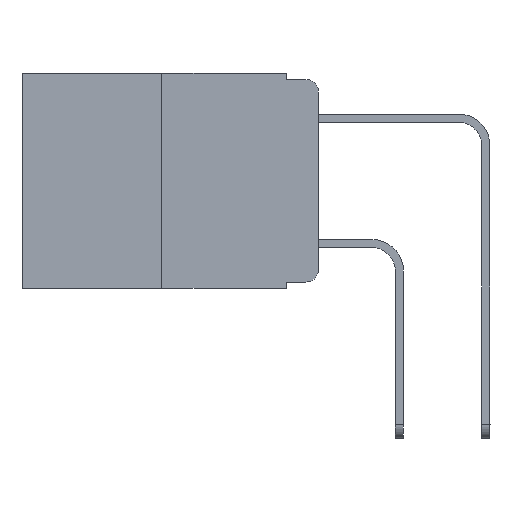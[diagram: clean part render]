
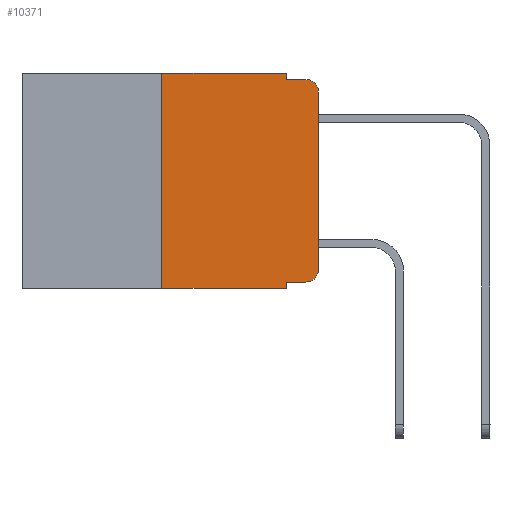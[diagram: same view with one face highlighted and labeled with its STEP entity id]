
A CAD part, left-side view. The second image highlights one B-rep face of the part: STEP entity #10371.
In plain terms, the highlighted planar face has unit normal (-1, 0, 0).
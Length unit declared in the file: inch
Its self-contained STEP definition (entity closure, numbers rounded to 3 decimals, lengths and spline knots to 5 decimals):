
#50 = CARTESIAN_POINT ( 'NONE',  ( 0., 0.02, -0.333 ) ) ;
#106 = DIRECTION ( 'NONE',  ( 0., 0., 1. ) ) ;
#331 = DIRECTION ( 'NONE',  ( 0., 0., -1. ) ) ;
#519 = LINE ( 'NONE', #2161, #13176 ) ;
#569 = DIRECTION ( 'NONE',  ( -1., 0., 0. ) ) ;
#697 = ORIENTED_EDGE ( 'NONE', *, *, #8291, .T. ) ;
#774 = LINE ( 'NONE', #5736, #8462 ) ;
#826 = ORIENTED_EDGE ( 'NONE', *, *, #14375, .T. ) ;
#1158 = EDGE_CURVE ( 'NONE', #8993, #12565, #5526, .T. ) ;
#1278 = ORIENTED_EDGE ( 'NONE', *, *, #1158, .F. ) ;
#1641 = PLANE ( 'NONE',  #4406 ) ;
#1923 = CARTESIAN_POINT ( 'NONE',  ( 0., 0.051, -0.333 ) ) ;
#2083 = VERTEX_POINT ( 'NONE', #13376 ) ;
#2118 = EDGE_CURVE ( 'NONE', #4404, #9830, #774, .T. ) ;
#2161 = CARTESIAN_POINT ( 'NONE',  ( 0., 0.473, -0.343 ) ) ;
#2166 = CARTESIAN_POINT ( 'NONE',  ( 0., 0.473, 0. ) ) ;
#2220 = ORIENTED_EDGE ( 'NONE', *, *, #2118, .F. ) ;
#2834 = EDGE_CURVE ( 'NONE', #12487, #8993, #9660, .T. ) ;
#2847 = EDGE_CURVE ( 'NONE', #10717, #12487, #7281, .T. ) ;
#3379 = CARTESIAN_POINT ( 'NONE',  ( 0., 0.051, 0. ) ) ;
#3672 = VECTOR ( 'NONE', #331, 39.37008 ) ;
#4078 = ORIENTED_EDGE ( 'NONE', *, *, #11253, .T. ) ;
#4216 = DIRECTION ( 'NONE',  ( 0., 0., -1. ) ) ;
#4354 = CARTESIAN_POINT ( 'NONE',  ( 0., 0.02, -0.313 ) ) ;
#4358 = CARTESIAN_POINT ( 'NONE',  ( 0., 0.051, 0. ) ) ;
#4399 = DIRECTION ( 'NONE',  ( 0., 0., -1. ) ) ;
#4404 = VERTEX_POINT ( 'NONE', #1923 ) ;
#4406 = AXIS2_PLACEMENT_3D ( 'NONE', #11532, #14225, #10143 ) ;
#4450 = CARTESIAN_POINT ( 'NONE',  ( 0., 0.051, -0.01 ) ) ;
#4464 = VECTOR ( 'NONE', #14658, 39.37008 ) ;
#4516 = EDGE_CURVE ( 'NONE', #13193, #6578, #13518, .T. ) ;
#4558 = LINE ( 'NONE', #13358, #4464 ) ;
#4631 = ORIENTED_EDGE ( 'NONE', *, *, #2847, .F. ) ;
#4706 = VECTOR ( 'NONE', #106, 39.37008 ) ;
#4885 = DIRECTION ( 'NONE',  ( 0., 0., 1. ) ) ;
#5056 = LINE ( 'NONE', #14007, #4706 ) ;
#5526 = LINE ( 'NONE', #4358, #3672 ) ;
#5600 = ORIENTED_EDGE ( 'NONE', *, *, #2834, .F. ) ;
#5615 = DIRECTION ( 'NONE',  ( 0., 0., -1. ) ) ;
#5736 = CARTESIAN_POINT ( 'NONE',  ( 0., 0.051, 0. ) ) ;
#5893 = VECTOR ( 'NONE', #5963, 39.37008 ) ;
#5963 = DIRECTION ( 'NONE',  ( 0., -1., 0. ) ) ;
#6080 = CARTESIAN_POINT ( 'NONE',  ( 0., 0.25, -0.343 ) ) ;
#6578 = VERTEX_POINT ( 'NONE', #12241 ) ;
#7051 = CARTESIAN_POINT ( 'NONE',  ( 0., 0.051, -0.343 ) ) ;
#7200 = DIRECTION ( 'NONE',  ( 0., -1., 0. ) ) ;
#7281 = LINE ( 'NONE', #8525, #16122 ) ;
#7855 = EDGE_LOOP ( 'NONE', ( #4078, #7937, #10215, #1278, #5600, #4631, #697, #2220, #10686, #826 ) ) ;
#7915 = CIRCLE ( 'NONE', #11060, 0.02 ) ;
#7937 = ORIENTED_EDGE ( 'NONE', *, *, #4516, .T. ) ;
#8265 = DIRECTION ( 'NONE',  ( -1., 0., 0. ) ) ;
#8291 = EDGE_CURVE ( 'NONE', #10717, #9830, #519, .T. ) ;
#8328 = EDGE_CURVE ( 'NONE', #4404, #9976, #4558, .T. ) ;
#8394 = VECTOR ( 'NONE', #10723, 39.37008 ) ;
#8462 = VECTOR ( 'NONE', #4399, 39.37008 ) ;
#8525 = CARTESIAN_POINT ( 'NONE',  ( 0., 0.25, 0. ) ) ;
#8993 = VERTEX_POINT ( 'NONE', #3379 ) ;
#9660 = LINE ( 'NONE', #2166, #5893 ) ;
#9830 = VERTEX_POINT ( 'NONE', #7051 ) ;
#9976 = VERTEX_POINT ( 'NONE', #50 ) ;
#10143 = DIRECTION ( 'NONE',  ( 0., 0., -1. ) ) ;
#10215 = ORIENTED_EDGE ( 'NONE', *, *, #11392, .F. ) ;
#10371 = ADVANCED_FACE ( 'NONE', ( #12683 ), #1641, .F. ) ;
#10686 = ORIENTED_EDGE ( 'NONE', *, *, #8328, .T. ) ;
#10717 = VERTEX_POINT ( 'NONE', #6080 ) ;
#10723 = DIRECTION ( 'NONE',  ( 0., -1., 0. ) ) ;
#10873 = CARTESIAN_POINT ( 'NONE',  ( 0., 0., -0.03 ) ) ;
#11060 = AXIS2_PLACEMENT_3D ( 'NONE', #4354, #569, #5615 ) ;
#11253 = EDGE_CURVE ( 'NONE', #2083, #13193, #5056, .T. ) ;
#11392 = EDGE_CURVE ( 'NONE', #12565, #6578, #14246, .T. ) ;
#11532 = CARTESIAN_POINT ( 'NONE',  ( 0., 0.473, 0. ) ) ;
#12241 = CARTESIAN_POINT ( 'NONE',  ( 0., 0.02, -0.01 ) ) ;
#12487 = VERTEX_POINT ( 'NONE', #12946 ) ;
#12565 = VERTEX_POINT ( 'NONE', #12862 ) ;
#12683 = FACE_OUTER_BOUND ( 'NONE', #7855, .T. ) ;
#12862 = CARTESIAN_POINT ( 'NONE',  ( 0., 0.051, -0.01 ) ) ;
#12946 = CARTESIAN_POINT ( 'NONE',  ( 0., 0.25, 0. ) ) ;
#13176 = VECTOR ( 'NONE', #7200, 39.37008 ) ;
#13193 = VERTEX_POINT ( 'NONE', #10873 ) ;
#13358 = CARTESIAN_POINT ( 'NONE',  ( 0., 0.051, -0.333 ) ) ;
#13376 = CARTESIAN_POINT ( 'NONE',  ( 0., 0., -0.313 ) ) ;
#13518 = CIRCLE ( 'NONE', #14300, 0.02 ) ;
#14007 = CARTESIAN_POINT ( 'NONE',  ( 0., 0., 0. ) ) ;
#14225 = DIRECTION ( 'NONE',  ( 1., 0., 0. ) ) ;
#14246 = LINE ( 'NONE', #4450, #8394 ) ;
#14300 = AXIS2_PLACEMENT_3D ( 'NONE', #14499, #8265, #4216 ) ;
#14375 = EDGE_CURVE ( 'NONE', #9976, #2083, #7915, .T. ) ;
#14499 = CARTESIAN_POINT ( 'NONE',  ( 0., 0.02, -0.03 ) ) ;
#14658 = DIRECTION ( 'NONE',  ( 0., -1., 0. ) ) ;
#16122 = VECTOR ( 'NONE', #4885, 39.37008 ) ;
